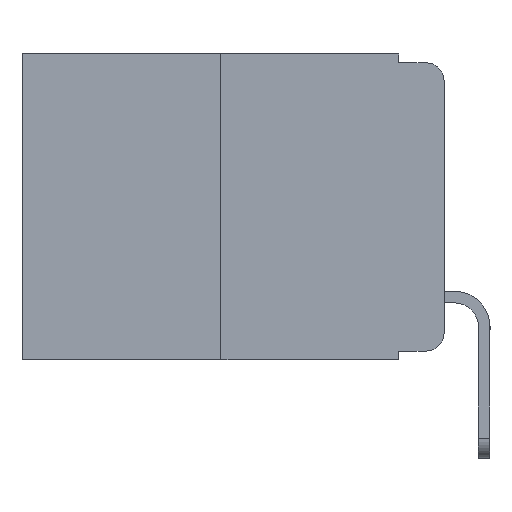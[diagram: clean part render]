
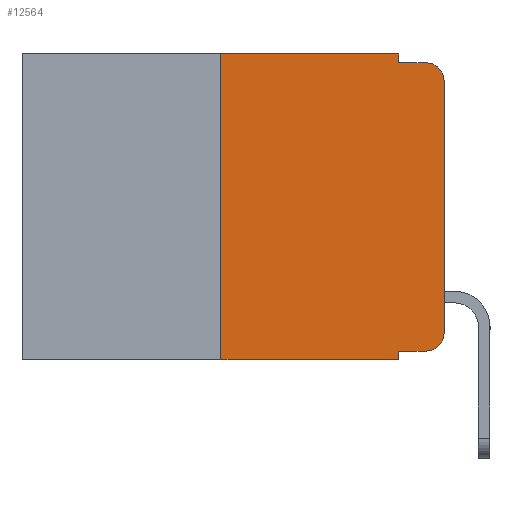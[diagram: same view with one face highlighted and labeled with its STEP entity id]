
A CAD part, left-side view. The second image highlights one B-rep face of the part: STEP entity #12564.
In plain terms, the highlighted planar face has unit normal (-1, 0, 0).
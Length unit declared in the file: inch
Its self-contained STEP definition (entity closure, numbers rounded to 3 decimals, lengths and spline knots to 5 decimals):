
#282 = DIRECTION ( 'NONE',  ( 0., 0., -1. ) ) ;
#406 = CARTESIAN_POINT ( 'NONE',  ( 0., 0.051, -0.01 ) ) ;
#603 = DIRECTION ( 'NONE',  ( -1., 0., 0. ) ) ;
#1106 = CARTESIAN_POINT ( 'NONE',  ( 0., 0.051, -0.343 ) ) ;
#1121 = DIRECTION ( 'NONE',  ( 0., 0., 1. ) ) ;
#1421 = CARTESIAN_POINT ( 'NONE',  ( 0., 0.25, 0. ) ) ;
#1640 = LINE ( 'NONE', #1901, #13454 ) ;
#1819 = AXIS2_PLACEMENT_3D ( 'NONE', #7560, #603, #8688 ) ;
#1869 = LINE ( 'NONE', #1421, #10464 ) ;
#1898 = LINE ( 'NONE', #13732, #4836 ) ;
#1901 = CARTESIAN_POINT ( 'NONE',  ( 0., 0.051, -0.01 ) ) ;
#2031 = ORIENTED_EDGE ( 'NONE', *, *, #6735, .F. ) ;
#2677 = DIRECTION ( 'NONE',  ( 0., 0., 1. ) ) ;
#2688 = EDGE_CURVE ( 'NONE', #9110, #7750, #12836, .T. ) ;
#2791 = VECTOR ( 'NONE', #10581, 39.37008 ) ;
#3347 = CARTESIAN_POINT ( 'NONE',  ( 0., 0., -0.313 ) ) ;
#3498 = AXIS2_PLACEMENT_3D ( 'NONE', #6400, #13957, #7506 ) ;
#3593 = PLANE ( 'NONE',  #12264 ) ;
#3625 = VECTOR ( 'NONE', #14309, 39.37008 ) ;
#3719 = CARTESIAN_POINT ( 'NONE',  ( 0., 0.051, -0.333 ) ) ;
#3730 = EDGE_CURVE ( 'NONE', #9110, #13284, #1869, .T. ) ;
#3865 = ORIENTED_EDGE ( 'NONE', *, *, #4762, .T. ) ;
#4265 = VERTEX_POINT ( 'NONE', #3347 ) ;
#4386 = ORIENTED_EDGE ( 'NONE', *, *, #13268, .T. ) ;
#4507 = VERTEX_POINT ( 'NONE', #3719 ) ;
#4762 = EDGE_CURVE ( 'NONE', #13412, #4265, #5806, .T. ) ;
#4836 = VECTOR ( 'NONE', #282, 39.37008 ) ;
#5028 = VERTEX_POINT ( 'NONE', #6875 ) ;
#5105 = CARTESIAN_POINT ( 'NONE',  ( 0., 0.051, 0. ) ) ;
#5570 = EDGE_CURVE ( 'NONE', #13284, #8878, #14132, .T. ) ;
#5631 = CARTESIAN_POINT ( 'NONE',  ( 0., 0.051, -0.333 ) ) ;
#5743 = VERTEX_POINT ( 'NONE', #8929 ) ;
#5790 = CARTESIAN_POINT ( 'NONE',  ( 0., 0.473, 0. ) ) ;
#5800 = ORIENTED_EDGE ( 'NONE', *, *, #5570, .F. ) ;
#5806 = CIRCLE ( 'NONE', #3498, 0.02 ) ;
#5811 = LINE ( 'NONE', #5105, #2791 ) ;
#5978 = EDGE_CURVE ( 'NONE', #8878, #14389, #5811, .T. ) ;
#6151 = ORIENTED_EDGE ( 'NONE', *, *, #2688, .T. ) ;
#6267 = DIRECTION ( 'NONE',  ( 0., -1., 0. ) ) ;
#6400 = CARTESIAN_POINT ( 'NONE',  ( 0., 0.02, -0.313 ) ) ;
#6596 = LINE ( 'NONE', #5631, #3625 ) ;
#6735 = EDGE_CURVE ( 'NONE', #14389, #5743, #1640, .T. ) ;
#6856 = EDGE_LOOP ( 'NONE', ( #4386, #10267, #2031, #14105, #5800, #14458, #6151, #9115, #12279, #3865 ) ) ;
#6875 = CARTESIAN_POINT ( 'NONE',  ( 0., 0., -0.03 ) ) ;
#6949 = DIRECTION ( 'NONE',  ( 0., 0., -1. ) ) ;
#7213 = CARTESIAN_POINT ( 'NONE',  ( 0., 0.051, 0. ) ) ;
#7506 = DIRECTION ( 'NONE',  ( 0., 0., -1. ) ) ;
#7560 = CARTESIAN_POINT ( 'NONE',  ( 0., 0.02, -0.03 ) ) ;
#7666 = CARTESIAN_POINT ( 'NONE',  ( 0., 0.25, -0.343 ) ) ;
#7750 = VERTEX_POINT ( 'NONE', #1106 ) ;
#7788 = FACE_OUTER_BOUND ( 'NONE', #6856, .T. ) ;
#8014 = CARTESIAN_POINT ( 'NONE',  ( 0., 0.25, 0. ) ) ;
#8432 = VECTOR ( 'NONE', #11755, 39.37008 ) ;
#8540 = CARTESIAN_POINT ( 'NONE',  ( 0., 0.473, 0. ) ) ;
#8688 = DIRECTION ( 'NONE',  ( 0., 0., -1. ) ) ;
#8878 = VERTEX_POINT ( 'NONE', #7213 ) ;
#8929 = CARTESIAN_POINT ( 'NONE',  ( 0., 0.02, -0.01 ) ) ;
#9110 = VERTEX_POINT ( 'NONE', #7666 ) ;
#9115 = ORIENTED_EDGE ( 'NONE', *, *, #12802, .F. ) ;
#9239 = EDGE_CURVE ( 'NONE', #4507, #13412, #6596, .T. ) ;
#9341 = CARTESIAN_POINT ( 'NONE',  ( 0., 0.02, -0.333 ) ) ;
#9541 = CARTESIAN_POINT ( 'NONE',  ( 0., 0.473, -0.343 ) ) ;
#9768 = DIRECTION ( 'NONE',  ( 0., -1., 0. ) ) ;
#10267 = ORIENTED_EDGE ( 'NONE', *, *, #10402, .T. ) ;
#10402 = EDGE_CURVE ( 'NONE', #5028, #5743, #11010, .T. ) ;
#10464 = VECTOR ( 'NONE', #2677, 39.37008 ) ;
#10581 = DIRECTION ( 'NONE',  ( 0., 0., -1. ) ) ;
#11010 = CIRCLE ( 'NONE', #1819, 0.02 ) ;
#11016 = VECTOR ( 'NONE', #1121, 39.37008 ) ;
#11348 = LINE ( 'NONE', #14453, #11016 ) ;
#11755 = DIRECTION ( 'NONE',  ( 0., -1., 0. ) ) ;
#12264 = AXIS2_PLACEMENT_3D ( 'NONE', #5790, #13429, #6949 ) ;
#12279 = ORIENTED_EDGE ( 'NONE', *, *, #9239, .T. ) ;
#12499 = VECTOR ( 'NONE', #6267, 39.37008 ) ;
#12564 = ADVANCED_FACE ( 'NONE', ( #7788 ), #3593, .F. ) ;
#12802 = EDGE_CURVE ( 'NONE', #4507, #7750, #1898, .T. ) ;
#12836 = LINE ( 'NONE', #9541, #12499 ) ;
#13268 = EDGE_CURVE ( 'NONE', #4265, #5028, #11348, .T. ) ;
#13284 = VERTEX_POINT ( 'NONE', #8014 ) ;
#13412 = VERTEX_POINT ( 'NONE', #9341 ) ;
#13429 = DIRECTION ( 'NONE',  ( 1., 0., 0. ) ) ;
#13454 = VECTOR ( 'NONE', #9768, 39.37008 ) ;
#13732 = CARTESIAN_POINT ( 'NONE',  ( 0., 0.051, 0. ) ) ;
#13957 = DIRECTION ( 'NONE',  ( -1., 0., 0. ) ) ;
#14105 = ORIENTED_EDGE ( 'NONE', *, *, #5978, .F. ) ;
#14132 = LINE ( 'NONE', #8540, #8432 ) ;
#14309 = DIRECTION ( 'NONE',  ( 0., -1., 0. ) ) ;
#14389 = VERTEX_POINT ( 'NONE', #406 ) ;
#14453 = CARTESIAN_POINT ( 'NONE',  ( 0., 0., 0. ) ) ;
#14458 = ORIENTED_EDGE ( 'NONE', *, *, #3730, .F. ) ;
